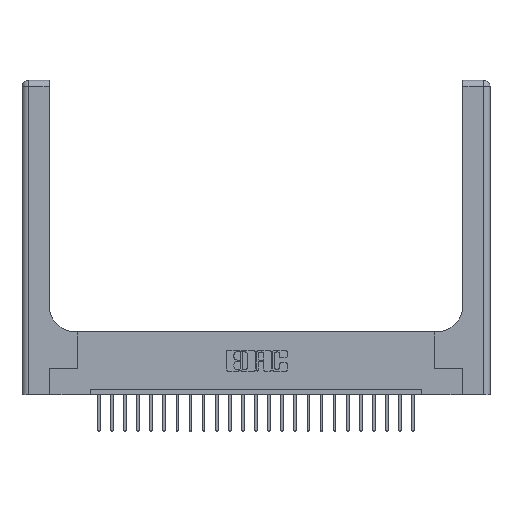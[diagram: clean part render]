
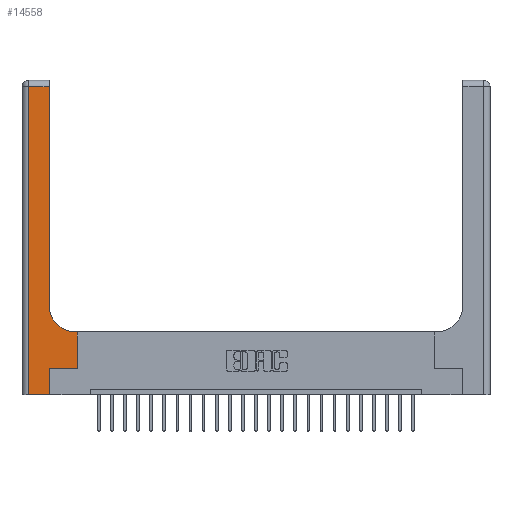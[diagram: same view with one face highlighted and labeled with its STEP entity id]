
A CAD part, top view. The second image highlights one B-rep face of the part: STEP entity #14558.
In plain terms, the highlighted planar face has unit normal (0, 0, 1).
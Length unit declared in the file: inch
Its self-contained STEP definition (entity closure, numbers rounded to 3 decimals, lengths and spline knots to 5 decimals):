
#592 = CARTESIAN_POINT ( 'NONE',  ( 0.528, 0.6, 0.37 ) ) ;
#661 = DIRECTION ( 'NONE',  ( 1., 0., 0. ) ) ;
#1176 = EDGE_CURVE ( 'NONE', #13216, #5842, #19910, .T. ) ;
#1204 = EDGE_CURVE ( 'NONE', #6877, #14274, #10776, .T. ) ;
#1798 = DIRECTION ( 'NONE',  ( 1., 0., 0. ) ) ;
#1822 = DIRECTION ( 'NONE',  ( 0., 1., 0. ) ) ;
#2228 = LINE ( 'NONE', #6841, #20820 ) ;
#2500 = VECTOR ( 'NONE', #20711, 39.37008 ) ;
#2539 = CARTESIAN_POINT ( 'NONE',  ( 0.265, 0., 0.37 ) ) ;
#2909 = FACE_OUTER_BOUND ( 'NONE', #19777, .T. ) ;
#3074 = ORIENTED_EDGE ( 'NONE', *, *, #5425, .T. ) ;
#3193 = VECTOR ( 'NONE', #20901, 39.37008 ) ;
#3536 = VECTOR ( 'NONE', #1822, 39.37008 ) ;
#4144 = VECTOR ( 'NONE', #12029, 39.37008 ) ;
#4713 = CARTESIAN_POINT ( 'NONE',  ( 0.265, 0., 0.37 ) ) ;
#4981 = EDGE_CURVE ( 'NONE', #18059, #6877, #9260, .T. ) ;
#5301 = ORIENTED_EDGE ( 'NONE', *, *, #14394, .T. ) ;
#5425 = EDGE_CURVE ( 'NONE', #5842, #18059, #11721, .T. ) ;
#5571 = CARTESIAN_POINT ( 'NONE',  ( 0., 3., 0.37 ) ) ;
#5842 = VERTEX_POINT ( 'NONE', #4713 ) ;
#5910 = ORIENTED_EDGE ( 'NONE', *, *, #4981, .T. ) ;
#5915 = VECTOR ( 'NONE', #16991, 39.37008 ) ;
#6460 = VECTOR ( 'NONE', #21803, 39.37008 ) ;
#6721 = CARTESIAN_POINT ( 'NONE',  ( 0.06, 2.94, 0.37 ) ) ;
#6841 = CARTESIAN_POINT ( 'NONE',  ( 0., 2.94, 0.37 ) ) ;
#6852 = CARTESIAN_POINT ( 'NONE',  ( 0.06, 3., 0.37 ) ) ;
#6877 = VERTEX_POINT ( 'NONE', #14717 ) ;
#7489 = LINE ( 'NONE', #6852, #4144 ) ;
#7904 = CARTESIAN_POINT ( 'NONE',  ( 0.26, 2.94, 0.37 ) ) ;
#8421 = AXIS2_PLACEMENT_3D ( 'NONE', #10533, #12455, #1798 ) ;
#8741 = CARTESIAN_POINT ( 'NONE',  ( 0.26, 3., 0.37 ) ) ;
#9221 = DIRECTION ( 'NONE',  ( 0., 0., -1. ) ) ;
#9260 = LINE ( 'NONE', #16915, #5915 ) ;
#9312 = ORIENTED_EDGE ( 'NONE', *, *, #11474, .T. ) ;
#9471 = EDGE_CURVE ( 'NONE', #14821, #11858, #14048, .T. ) ;
#9533 = CARTESIAN_POINT ( 'NONE',  ( 0., 0., 0.37 ) ) ;
#9905 = LINE ( 'NONE', #8741, #3193 ) ;
#10533 = CARTESIAN_POINT ( 'NONE',  ( 0.51, 0.85, 0.37 ) ) ;
#10584 = CARTESIAN_POINT ( 'NONE',  ( 0.265, 0.25, 0.37 ) ) ;
#10776 = LINE ( 'NONE', #15953, #3536 ) ;
#11099 = DIRECTION ( 'NONE',  ( -1., 0., 0. ) ) ;
#11394 = EDGE_CURVE ( 'NONE', #15914, #18871, #2228, .T. ) ;
#11474 = EDGE_CURVE ( 'NONE', #14274, #14821, #19986, .T. ) ;
#11721 = LINE ( 'NONE', #2539, #6460 ) ;
#11858 = VERTEX_POINT ( 'NONE', #19256 ) ;
#12029 = DIRECTION ( 'NONE',  ( 0., -1., 0. ) ) ;
#12455 = DIRECTION ( 'NONE',  ( 0., 0., -1. ) ) ;
#13214 = ORIENTED_EDGE ( 'NONE', *, *, #18476, .T. ) ;
#13216 = VERTEX_POINT ( 'NONE', #18531 ) ;
#13477 = ORIENTED_EDGE ( 'NONE', *, *, #11394, .T. ) ;
#14048 = CIRCLE ( 'NONE', #8421, 0.25 ) ;
#14274 = VERTEX_POINT ( 'NONE', #592 ) ;
#14394 = EDGE_CURVE ( 'NONE', #11858, #15914, #9905, .T. ) ;
#14558 = ADVANCED_FACE ( 'NONE', ( #2909 ), #21698, .F. ) ;
#14717 = CARTESIAN_POINT ( 'NONE',  ( 0.528, 0.25, 0.37 ) ) ;
#14821 = VERTEX_POINT ( 'NONE', #18122 ) ;
#15622 = ORIENTED_EDGE ( 'NONE', *, *, #9471, .T. ) ;
#15914 = VERTEX_POINT ( 'NONE', #7904 ) ;
#15953 = CARTESIAN_POINT ( 'NONE',  ( 0.528, 0.25, 0.37 ) ) ;
#16915 = CARTESIAN_POINT ( 'NONE',  ( 0.265, 0.25, 0.37 ) ) ;
#16991 = DIRECTION ( 'NONE',  ( 1., 0., 0. ) ) ;
#17125 = VECTOR ( 'NONE', #661, 39.37008 ) ;
#18059 = VERTEX_POINT ( 'NONE', #10584 ) ;
#18122 = CARTESIAN_POINT ( 'NONE',  ( 0.51, 0.6, 0.37 ) ) ;
#18394 = AXIS2_PLACEMENT_3D ( 'NONE', #5571, #9221, #11099 ) ;
#18476 = EDGE_CURVE ( 'NONE', #18871, #13216, #7489, .T. ) ;
#18531 = CARTESIAN_POINT ( 'NONE',  ( 0.06, 0., 0.37 ) ) ;
#18871 = VERTEX_POINT ( 'NONE', #6721 ) ;
#19256 = CARTESIAN_POINT ( 'NONE',  ( 0.26, 0.85, 0.37 ) ) ;
#19557 = ORIENTED_EDGE ( 'NONE', *, *, #1176, .T. ) ;
#19585 = ORIENTED_EDGE ( 'NONE', *, *, #1204, .T. ) ;
#19777 = EDGE_LOOP ( 'NONE', ( #5301, #13477, #13214, #19557, #3074, #5910, #19585, #9312, #15622 ) ) ;
#19910 = LINE ( 'NONE', #9533, #17125 ) ;
#19986 = LINE ( 'NONE', #20861, #2500 ) ;
#20711 = DIRECTION ( 'NONE',  ( -1., 0., 0. ) ) ;
#20790 = DIRECTION ( 'NONE',  ( -1., 0., 0. ) ) ;
#20820 = VECTOR ( 'NONE', #20790, 39.37008 ) ;
#20861 = CARTESIAN_POINT ( 'NONE',  ( 0.26, 0.6, 0.37 ) ) ;
#20901 = DIRECTION ( 'NONE',  ( 0., 1., 0. ) ) ;
#21698 = PLANE ( 'NONE',  #18394 ) ;
#21803 = DIRECTION ( 'NONE',  ( 0., 1., 0. ) ) ;
